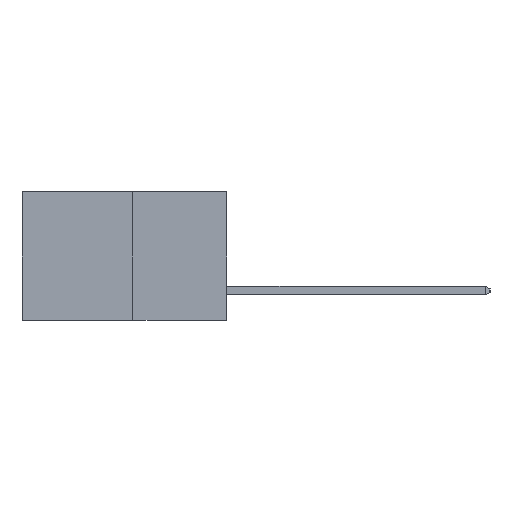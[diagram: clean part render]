
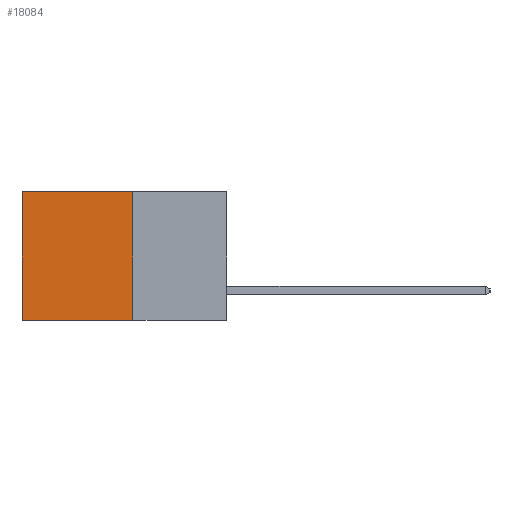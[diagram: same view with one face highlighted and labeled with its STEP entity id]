
A CAD part, left-side view. The second image highlights one B-rep face of the part: STEP entity #18084.
In plain terms, the highlighted planar face has unit normal (-1, 0, 0).
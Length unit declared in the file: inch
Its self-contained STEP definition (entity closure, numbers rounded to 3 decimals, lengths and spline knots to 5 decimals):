
#505 = ORIENTED_EDGE ( 'NONE', *, *, #20733, .F. ) ;
#2782 = CARTESIAN_POINT ( 'NONE',  ( 0.277, 0.27, -0.37 ) ) ;
#3220 = CARTESIAN_POINT ( 'NONE',  ( 0.277, 0.59, -0.37 ) ) ;
#4559 = ORIENTED_EDGE ( 'NONE', *, *, #6604, .T. ) ;
#5196 = CARTESIAN_POINT ( 'NONE',  ( 0.277, 0.27, -0.37 ) ) ;
#5606 = AXIS2_PLACEMENT_3D ( 'NONE', #2782, #9272, #20381 ) ;
#5618 = CARTESIAN_POINT ( 'NONE',  ( 0.277, 0.59, -0.37 ) ) ;
#5819 = DIRECTION ( 'NONE',  ( 0., 0., -1. ) ) ;
#6461 = DIRECTION ( 'NONE',  ( 0., 0., -1. ) ) ;
#6604 = EDGE_CURVE ( 'NONE', #7372, #12420, #11878, .T. ) ;
#6851 = CARTESIAN_POINT ( 'NONE',  ( 0.277, 0.27, -0.37 ) ) ;
#7372 = VERTEX_POINT ( 'NONE', #13011 ) ;
#7839 = LINE ( 'NONE', #9005, #15372 ) ;
#8466 = DIRECTION ( 'NONE',  ( 0., 1., 0. ) ) ;
#8468 = EDGE_LOOP ( 'NONE', ( #15486, #9782, #505, #4559 ) ) ;
#9005 = CARTESIAN_POINT ( 'NONE',  ( 0.277, 0.27, -0.37 ) ) ;
#9212 = CARTESIAN_POINT ( 'NONE',  ( 0.277, 0.27, 0. ) ) ;
#9272 = DIRECTION ( 'NONE',  ( 1., 0., 0. ) ) ;
#9375 = FACE_OUTER_BOUND ( 'NONE', #8468, .T. ) ;
#9782 = ORIENTED_EDGE ( 'NONE', *, *, #12275, .F. ) ;
#10778 = LINE ( 'NONE', #3220, #18729 ) ;
#11390 = VECTOR ( 'NONE', #12463, 39.37008 ) ;
#11579 = EDGE_CURVE ( 'NONE', #12420, #20655, #10778, .T. ) ;
#11878 = LINE ( 'NONE', #9212, #11390 ) ;
#12275 = EDGE_CURVE ( 'NONE', #17717, #20655, #13548, .T. ) ;
#12420 = VERTEX_POINT ( 'NONE', #15135 ) ;
#12463 = DIRECTION ( 'NONE',  ( 0., 1., 0. ) ) ;
#13011 = CARTESIAN_POINT ( 'NONE',  ( 0.277, 0.27, 0. ) ) ;
#13548 = LINE ( 'NONE', #6851, #18245 ) ;
#15135 = CARTESIAN_POINT ( 'NONE',  ( 0.277, 0.59, 0. ) ) ;
#15372 = VECTOR ( 'NONE', #5819, 39.37008 ) ;
#15486 = ORIENTED_EDGE ( 'NONE', *, *, #11579, .T. ) ;
#17717 = VERTEX_POINT ( 'NONE', #5196 ) ;
#18084 = ADVANCED_FACE ( 'NONE', ( #9375 ), #18814, .F. ) ;
#18245 = VECTOR ( 'NONE', #8466, 39.37008 ) ;
#18729 = VECTOR ( 'NONE', #6461, 39.37008 ) ;
#18814 = PLANE ( 'NONE',  #5606 ) ;
#20381 = DIRECTION ( 'NONE',  ( 0., 0., -1. ) ) ;
#20655 = VERTEX_POINT ( 'NONE', #5618 ) ;
#20733 = EDGE_CURVE ( 'NONE', #7372, #17717, #7839, .T. ) ;
